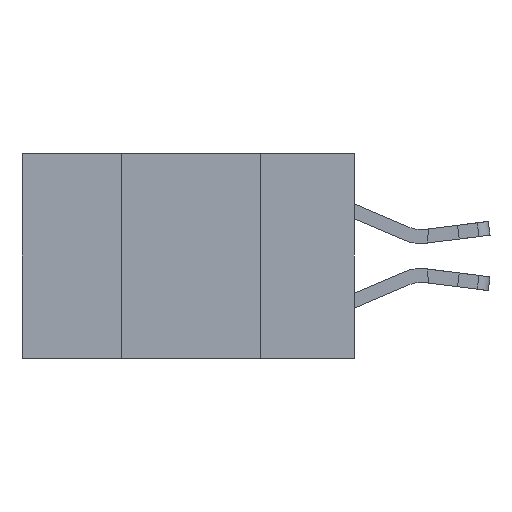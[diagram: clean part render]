
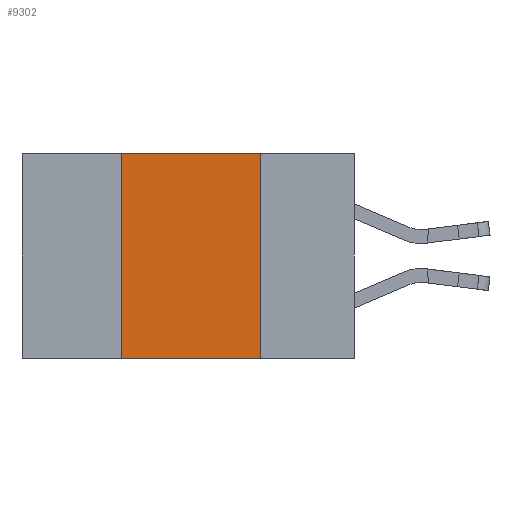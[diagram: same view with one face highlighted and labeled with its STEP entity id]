
A CAD part, left-side view. The second image highlights one B-rep face of the part: STEP entity #9302.
In plain terms, the highlighted planar face has unit normal (-1, 0, 0).
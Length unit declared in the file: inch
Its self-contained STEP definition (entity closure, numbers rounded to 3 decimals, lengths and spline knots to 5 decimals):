
#416 = LINE ( 'NONE', #11524, #7045 ) ;
#682 = ORIENTED_EDGE ( 'NONE', *, *, #14690, .F. ) ;
#764 = VERTEX_POINT ( 'NONE', #19403 ) ;
#1807 = LINE ( 'NONE', #17231, #12130 ) ;
#1903 = EDGE_CURVE ( 'NONE', #20372, #19761, #1807, .T. ) ;
#2138 = CARTESIAN_POINT ( 'NONE',  ( 0., 0.17, -0.37 ) ) ;
#4079 = LINE ( 'NONE', #2138, #17020 ) ;
#4123 = CARTESIAN_POINT ( 'NONE',  ( 0., 0.6, 0. ) ) ;
#5284 = DIRECTION ( 'NONE',  ( 0., -1., 0. ) ) ;
#5585 = PLANE ( 'NONE',  #8623 ) ;
#7045 = VECTOR ( 'NONE', #5284, 39.37008 ) ;
#8623 = AXIS2_PLACEMENT_3D ( 'NONE', #4123, #10653, #15131 ) ;
#8913 = ORIENTED_EDGE ( 'NONE', *, *, #1903, .T. ) ;
#9302 = ADVANCED_FACE ( 'NONE', ( #18545 ), #5585, .F. ) ;
#9923 = VERTEX_POINT ( 'NONE', #18318 ) ;
#10533 = CARTESIAN_POINT ( 'NONE',  ( 0., 0.17, -0.37 ) ) ;
#10653 = DIRECTION ( 'NONE',  ( 1., 0., 0. ) ) ;
#10737 = DIRECTION ( 'NONE',  ( 0., 0., 1. ) ) ;
#11524 = CARTESIAN_POINT ( 'NONE',  ( 0., 0.6, 0. ) ) ;
#12074 = DIRECTION ( 'NONE',  ( 0., 0., -1. ) ) ;
#12130 = VECTOR ( 'NONE', #17345, 39.37008 ) ;
#12304 = LINE ( 'NONE', #18838, #12408 ) ;
#12408 = VECTOR ( 'NONE', #10737, 39.37008 ) ;
#13642 = EDGE_CURVE ( 'NONE', #764, #9923, #416, .T. ) ;
#14690 = EDGE_CURVE ( 'NONE', #9923, #19761, #4079, .T. ) ;
#15131 = DIRECTION ( 'NONE',  ( 0., 0., -1. ) ) ;
#15789 = EDGE_CURVE ( 'NONE', #20372, #764, #12304, .T. ) ;
#17020 = VECTOR ( 'NONE', #12074, 39.37008 ) ;
#17231 = CARTESIAN_POINT ( 'NONE',  ( 0., 0.6, -0.37 ) ) ;
#17248 = EDGE_LOOP ( 'NONE', ( #682, #18206, #17879, #8913 ) ) ;
#17345 = DIRECTION ( 'NONE',  ( 0., -1., 0. ) ) ;
#17879 = ORIENTED_EDGE ( 'NONE', *, *, #15789, .F. ) ;
#18206 = ORIENTED_EDGE ( 'NONE', *, *, #13642, .F. ) ;
#18318 = CARTESIAN_POINT ( 'NONE',  ( 0., 0.17, 0. ) ) ;
#18545 = FACE_OUTER_BOUND ( 'NONE', #17248, .T. ) ;
#18838 = CARTESIAN_POINT ( 'NONE',  ( 0., 0.42, -0.37 ) ) ;
#19117 = CARTESIAN_POINT ( 'NONE',  ( 0., 0.42, -0.37 ) ) ;
#19403 = CARTESIAN_POINT ( 'NONE',  ( 0., 0.42, 0. ) ) ;
#19761 = VERTEX_POINT ( 'NONE', #10533 ) ;
#20372 = VERTEX_POINT ( 'NONE', #19117 ) ;
